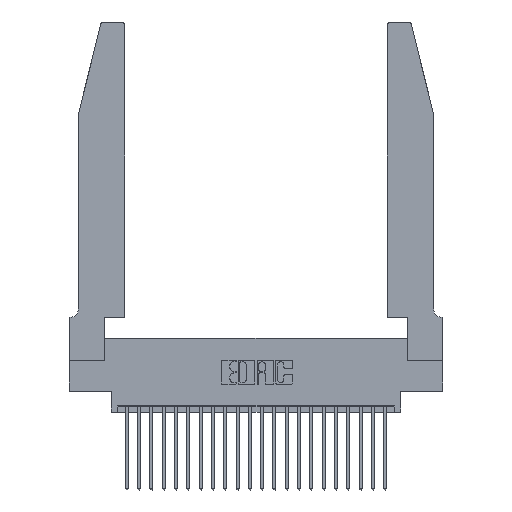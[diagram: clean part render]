
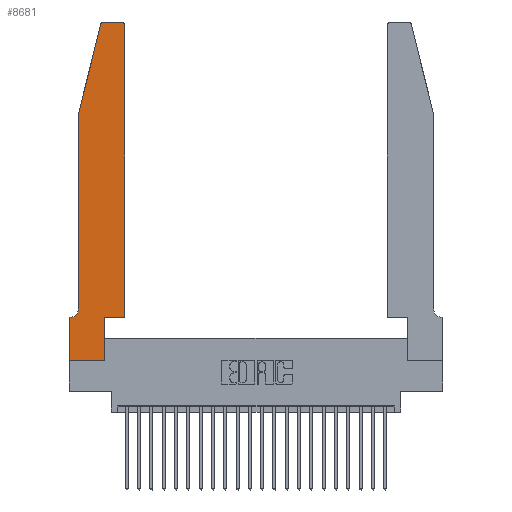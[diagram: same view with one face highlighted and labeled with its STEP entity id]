
A CAD part, top view. The second image highlights one B-rep face of the part: STEP entity #8681.
In plain terms, the highlighted planar face has unit normal (0, 0, 1).
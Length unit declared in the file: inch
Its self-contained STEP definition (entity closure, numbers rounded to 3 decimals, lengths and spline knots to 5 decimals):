
#117 = EDGE_LOOP ( 'NONE', ( #6655, #19545, #22034, #5505, #18372, #9685, #11114, #6213, #4225, #20785, #14357, #2888 ) ) ;
#272 = VERTEX_POINT ( 'NONE', #8565 ) ;
#518 = CARTESIAN_POINT ( 'NONE',  ( 0.0755, 2., 0.37 ) ) ;
#1022 = CARTESIAN_POINT ( 'NONE',  ( 0.2605, 2.75, 0.37 ) ) ;
#1060 = DIRECTION ( 'NONE',  ( 1., 0., 0. ) ) ;
#1098 = DIRECTION ( 'NONE',  ( -1., 0., 0. ) ) ;
#1329 = CARTESIAN_POINT ( 'NONE',  ( 0.284, 2.72, 0.37 ) ) ;
#2048 = CARTESIAN_POINT ( 'NONE',  ( 0., 0., 0.37 ) ) ;
#2163 = LINE ( 'NONE', #17075, #16981 ) ;
#2237 = CARTESIAN_POINT ( 'NONE',  ( 0.4505, 2.72, 0.37 ) ) ;
#2475 = CARTESIAN_POINT ( 'NONE',  ( 0., 0., 0.37 ) ) ;
#2888 = ORIENTED_EDGE ( 'NONE', *, *, #23847, .T. ) ;
#3150 = CARTESIAN_POINT ( 'NONE',  ( 0.0755, 2., 0.37 ) ) ;
#3364 = DIRECTION ( 'NONE',  ( 1., 0., 0. ) ) ;
#3612 = EDGE_CURVE ( 'NONE', #6255, #11026, #12575, .T. ) ;
#3643 = VECTOR ( 'NONE', #5655, 39.37008 ) ;
#3698 = DIRECTION ( 'NONE',  ( 1., 0., 0. ) ) ;
#3722 = EDGE_CURVE ( 'NONE', #6345, #272, #10754, .T. ) ;
#4225 = ORIENTED_EDGE ( 'NONE', *, *, #3722, .T. ) ;
#4510 = DIRECTION ( 'NONE',  ( 0., 0., -1. ) ) ;
#4707 = LINE ( 'NONE', #16639, #19992 ) ;
#4812 = CARTESIAN_POINT ( 'NONE',  ( 0.0055, 0.35, 0.37 ) ) ;
#5505 = ORIENTED_EDGE ( 'NONE', *, *, #22849, .T. ) ;
#5655 = DIRECTION ( 'NONE',  ( 1., 0., 0. ) ) ;
#5904 = VERTEX_POINT ( 'NONE', #17593 ) ;
#5908 = VERTEX_POINT ( 'NONE', #2237 ) ;
#5941 = AXIS2_PLACEMENT_3D ( 'NONE', #16196, #10523, #23700 ) ;
#6200 = CIRCLE ( 'NONE', #8517, 0.07 ) ;
#6213 = ORIENTED_EDGE ( 'NONE', *, *, #15000, .T. ) ;
#6255 = VERTEX_POINT ( 'NONE', #15046 ) ;
#6345 = VERTEX_POINT ( 'NONE', #15211 ) ;
#6617 = VERTEX_POINT ( 'NONE', #2475 ) ;
#6641 = EDGE_CURVE ( 'NONE', #19677, #22011, #6200, .T. ) ;
#6655 = ORIENTED_EDGE ( 'NONE', *, *, #3612, .T. ) ;
#7167 = EDGE_CURVE ( 'NONE', #13663, #5908, #19063, .T. ) ;
#7321 = CARTESIAN_POINT ( 'NONE',  ( 0.2865, 0.35, 0.37 ) ) ;
#7437 = AXIS2_PLACEMENT_3D ( 'NONE', #1329, #14975, #3364 ) ;
#7532 = LINE ( 'NONE', #2048, #17122 ) ;
#7604 = CIRCLE ( 'NONE', #19467, 0.03 ) ;
#8222 = LINE ( 'NONE', #19065, #3643 ) ;
#8517 = AXIS2_PLACEMENT_3D ( 'NONE', #16102, #4510, #17968 ) ;
#8565 = CARTESIAN_POINT ( 'NONE',  ( 0.2865, 0.35, 0.37 ) ) ;
#8571 = PLANE ( 'NONE',  #5941 ) ;
#8681 = ADVANCED_FACE ( 'NONE', ( #11608 ), #8571, .T. ) ;
#9012 = CARTESIAN_POINT ( 'NONE',  ( 0.0755, 0.42, 0.37 ) ) ;
#9589 = VERTEX_POINT ( 'NONE', #10037 ) ;
#9685 = ORIENTED_EDGE ( 'NONE', *, *, #20862, .T. ) ;
#10037 = CARTESIAN_POINT ( 'NONE',  ( 0.25487, 2.72718, 0.37 ) ) ;
#10523 = DIRECTION ( 'NONE',  ( 0., 0., 1. ) ) ;
#10754 = LINE ( 'NONE', #7321, #15226 ) ;
#11026 = VERTEX_POINT ( 'NONE', #13664 ) ;
#11114 = ORIENTED_EDGE ( 'NONE', *, *, #16444, .T. ) ;
#11608 = FACE_OUTER_BOUND ( 'NONE', #117, .T. ) ;
#12324 = DIRECTION ( 'NONE',  ( -0.239, -0.971, 0. ) ) ;
#12575 = LINE ( 'NONE', #1022, #21975 ) ;
#12835 = DIRECTION ( 'NONE',  ( 0., 0., 1. ) ) ;
#13615 = VERTEX_POINT ( 'NONE', #22159 ) ;
#13663 = VERTEX_POINT ( 'NONE', #14854 ) ;
#13664 = CARTESIAN_POINT ( 'NONE',  ( 0.284, 2.75, 0.37 ) ) ;
#13938 = CARTESIAN_POINT ( 'NONE',  ( 0.4505, 0.35, 0.37 ) ) ;
#14357 = ORIENTED_EDGE ( 'NONE', *, *, #7167, .T. ) ;
#14854 = CARTESIAN_POINT ( 'NONE',  ( 0.4505, 0.35, 0.37 ) ) ;
#14975 = DIRECTION ( 'NONE',  ( 0., 0., 1. ) ) ;
#15000 = EDGE_CURVE ( 'NONE', #6617, #6345, #8222, .T. ) ;
#15046 = CARTESIAN_POINT ( 'NONE',  ( 0.4205, 2.75, 0.37 ) ) ;
#15205 = VECTOR ( 'NONE', #24087, 39.37008 ) ;
#15211 = CARTESIAN_POINT ( 'NONE',  ( 0.2865, 0., 0.37 ) ) ;
#15226 = VECTOR ( 'NONE', #20648, 39.37008 ) ;
#15624 = DIRECTION ( 'NONE',  ( 0., -1., 0. ) ) ;
#16102 = CARTESIAN_POINT ( 'NONE',  ( 0.0055, 0.42, 0.37 ) ) ;
#16196 = CARTESIAN_POINT ( 'NONE',  ( 0., 0.35, 0.37 ) ) ;
#16391 = LINE ( 'NONE', #3150, #15205 ) ;
#16437 = VECTOR ( 'NONE', #12324, 39.37008 ) ;
#16444 = EDGE_CURVE ( 'NONE', #5904, #6617, #7532, .T. ) ;
#16460 = CIRCLE ( 'NONE', #7437, 0.03 ) ;
#16639 = CARTESIAN_POINT ( 'NONE',  ( 0.0755, 0.35, 0.37 ) ) ;
#16981 = VECTOR ( 'NONE', #3698, 39.37008 ) ;
#17075 = CARTESIAN_POINT ( 'NONE',  ( 0.4505, 0.35, 0.37 ) ) ;
#17122 = VECTOR ( 'NONE', #15624, 39.37008 ) ;
#17593 = CARTESIAN_POINT ( 'NONE',  ( 0., 0.35, 0.37 ) ) ;
#17698 = DIRECTION ( 'NONE',  ( 0., 1., 0. ) ) ;
#17968 = DIRECTION ( 'NONE',  ( -1., 0., 0. ) ) ;
#18372 = ORIENTED_EDGE ( 'NONE', *, *, #6641, .T. ) ;
#19063 = LINE ( 'NONE', #13938, #24021 ) ;
#19065 = CARTESIAN_POINT ( 'NONE',  ( 0., 0., 0.37 ) ) ;
#19467 = AXIS2_PLACEMENT_3D ( 'NONE', #24044, #12835, #1060 ) ;
#19545 = ORIENTED_EDGE ( 'NONE', *, *, #21474, .T. ) ;
#19677 = VERTEX_POINT ( 'NONE', #9012 ) ;
#19992 = VECTOR ( 'NONE', #1098, 39.37008 ) ;
#20648 = DIRECTION ( 'NONE',  ( 0., 1., 0. ) ) ;
#20785 = ORIENTED_EDGE ( 'NONE', *, *, #22320, .T. ) ;
#20862 = EDGE_CURVE ( 'NONE', #22011, #5904, #4707, .T. ) ;
#21389 = LINE ( 'NONE', #518, #16437 ) ;
#21474 = EDGE_CURVE ( 'NONE', #11026, #9589, #16460, .T. ) ;
#21926 = EDGE_CURVE ( 'NONE', #9589, #13615, #21389, .T. ) ;
#21975 = VECTOR ( 'NONE', #22145, 39.37008 ) ;
#22011 = VERTEX_POINT ( 'NONE', #4812 ) ;
#22034 = ORIENTED_EDGE ( 'NONE', *, *, #21926, .T. ) ;
#22145 = DIRECTION ( 'NONE',  ( -1., 0., 0. ) ) ;
#22159 = CARTESIAN_POINT ( 'NONE',  ( 0.0755, 2., 0.37 ) ) ;
#22320 = EDGE_CURVE ( 'NONE', #272, #13663, #2163, .T. ) ;
#22849 = EDGE_CURVE ( 'NONE', #13615, #19677, #16391, .T. ) ;
#23700 = DIRECTION ( 'NONE',  ( 1., 0., 0. ) ) ;
#23847 = EDGE_CURVE ( 'NONE', #5908, #6255, #7604, .T. ) ;
#24021 = VECTOR ( 'NONE', #17698, 39.37008 ) ;
#24044 = CARTESIAN_POINT ( 'NONE',  ( 0.4205, 2.72, 0.37 ) ) ;
#24087 = DIRECTION ( 'NONE',  ( 0., -1., 0. ) ) ;
